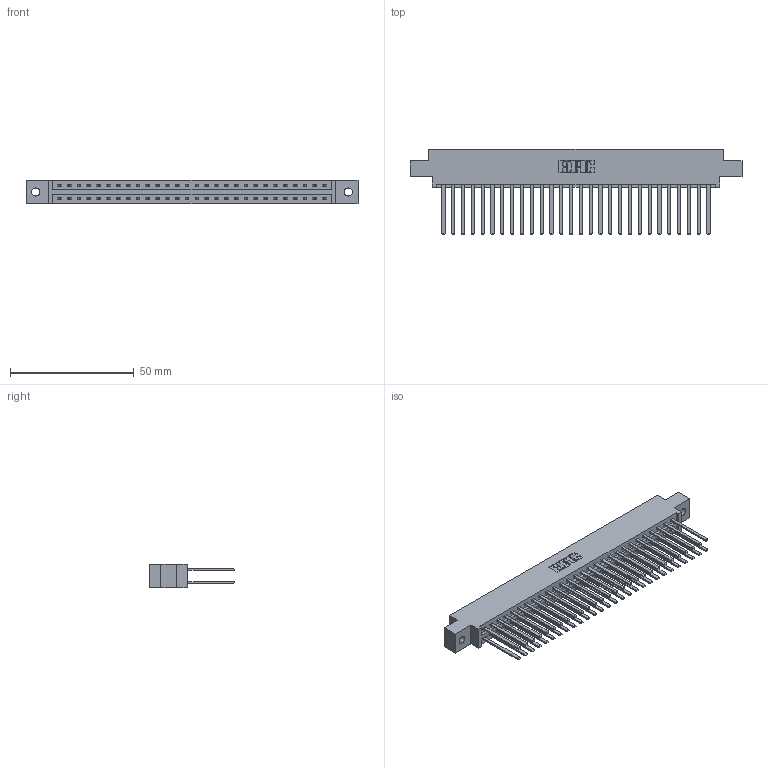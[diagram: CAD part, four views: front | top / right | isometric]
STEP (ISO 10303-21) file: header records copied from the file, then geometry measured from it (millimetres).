
FILE_DESCRIPTION (( 'STEP AP203' ), '1' );
FILE_NAME ('387-056-544-802.STEP', '2019-10-19T07:20:27', ( '' ), ( '' ), 'SwSTEP 2.0', 'SolidWorks 2016', '' );
FILE_SCHEMA (( 'CONFIG_CONTROL_DESIGN' ));
Length unit declared in the file: inch
Products named in the file (3): 345-292-001_345-293-144; 337 Part_0.170 Offset - 0.128 Dia; 387-056-544-802
Assembly tree (57 placements, depth 2):
  387-056-544-802
    337 Part_0.170 Offset - 0.128 Dia
    345-292-001_345-293-144  x56
Bounding box: 133.96 x 34.3 x 9.4 mm (x, y, z)
Volume: 14562.2 mm3; surface area: 18726.2 mm2
Topology: 57 solids, 57 shells, 2806 faces, 8331 edges, 5478 vertices
Faces by surface type: plane 1978, cylinder 828
Entity records: 23471 total; most frequent: CARTESIAN_POINT 3966, ORIENTED_EDGE 3902, DIRECTION 3395, EDGE_CURVE 1951, LINE 1827, VECTOR 1827, VERTEX_POINT 1298, AXIS2_PLACEMENT_3D 784
